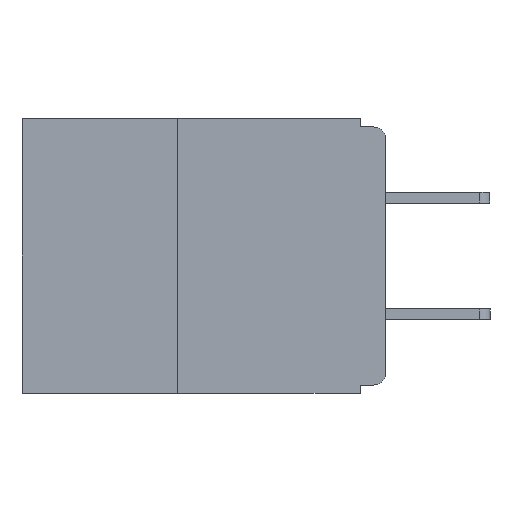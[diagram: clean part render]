
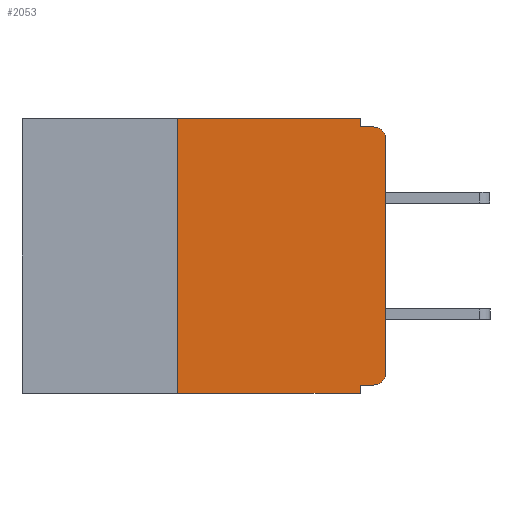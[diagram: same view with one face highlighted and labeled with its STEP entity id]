
A CAD part, left-side view. The second image highlights one B-rep face of the part: STEP entity #2053.
In plain terms, the highlighted planar face has unit normal (-1, 0, 0).
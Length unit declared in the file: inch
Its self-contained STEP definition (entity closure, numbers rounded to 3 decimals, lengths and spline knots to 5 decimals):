
#310 = DIRECTION ( 'NONE',  ( 0., 0., -1. ) ) ;
#402 = LINE ( 'NONE', #18275, #13644 ) ;
#642 = CIRCLE ( 'NONE', #13474, 0.015 ) ;
#1498 = AXIS2_PLACEMENT_3D ( 'NONE', #13234, #32510, #16109 ) ;
#2053 = ADVANCED_FACE ( 'NONE', ( #9263 ), #13210, .F. ) ;
#2341 = LINE ( 'NONE', #31891, #8912 ) ;
#2536 = ORIENTED_EDGE ( 'NONE', *, *, #6000, .F. ) ;
#2590 = ORIENTED_EDGE ( 'NONE', *, *, #15401, .F. ) ;
#2752 = CARTESIAN_POINT ( 'NONE',  ( 0., 0.25, -0.33 ) ) ;
#2807 = EDGE_CURVE ( 'NONE', #19424, #23672, #13187, .T. ) ;
#2842 = DIRECTION ( 'NONE',  ( 0., -1., 0. ) ) ;
#2897 = VERTEX_POINT ( 'NONE', #19834 ) ;
#3259 = VERTEX_POINT ( 'NONE', #11582 ) ;
#3335 = CARTESIAN_POINT ( 'NONE',  ( 0., 0., -0.305 ) ) ;
#3467 = CARTESIAN_POINT ( 'NONE',  ( 0., 0.437, -0.33 ) ) ;
#3662 = VERTEX_POINT ( 'NONE', #31116 ) ;
#3770 = LINE ( 'NONE', #13402, #25212 ) ;
#5061 = CARTESIAN_POINT ( 'NONE',  ( 0., 0.031, 0. ) ) ;
#5677 = EDGE_CURVE ( 'NONE', #13860, #12004, #34432, .T. ) ;
#6000 = EDGE_CURVE ( 'NONE', #2897, #26076, #16942, .T. ) ;
#6539 = ORIENTED_EDGE ( 'NONE', *, *, #5677, .T. ) ;
#6686 = EDGE_CURVE ( 'NONE', #26076, #3662, #2341, .T. ) ;
#7428 = LINE ( 'NONE', #5061, #35786 ) ;
#8818 = CARTESIAN_POINT ( 'NONE',  ( 0., 0.25, 0. ) ) ;
#8912 = VECTOR ( 'NONE', #31940, 39.37008 ) ;
#9180 = VERTEX_POINT ( 'NONE', #24794 ) ;
#9263 = FACE_OUTER_BOUND ( 'NONE', #31676, .T. ) ;
#9304 = ORIENTED_EDGE ( 'NONE', *, *, #29555, .F. ) ;
#9795 = EDGE_CURVE ( 'NONE', #3259, #20305, #7428, .T. ) ;
#10365 = EDGE_CURVE ( 'NONE', #19424, #3662, #18882, .T. ) ;
#11582 = CARTESIAN_POINT ( 'NONE',  ( 0., 0.031, 0. ) ) ;
#12004 = VERTEX_POINT ( 'NONE', #19621 ) ;
#12491 = EDGE_CURVE ( 'NONE', #12004, #9180, #22993, .T. ) ;
#13187 = LINE ( 'NONE', #21651, #27131 ) ;
#13210 = PLANE ( 'NONE',  #24238 ) ;
#13234 = CARTESIAN_POINT ( 'NONE',  ( 0., 0.015, -0.025 ) ) ;
#13293 = DIRECTION ( 'NONE',  ( 0., 0., -1. ) ) ;
#13402 = CARTESIAN_POINT ( 'NONE',  ( 0., 0., -0.01 ) ) ;
#13474 = AXIS2_PLACEMENT_3D ( 'NONE', #33590, #17268, #310 ) ;
#13644 = VECTOR ( 'NONE', #31937, 39.37008 ) ;
#13733 = CARTESIAN_POINT ( 'NONE',  ( 0., 0.031, -0.32 ) ) ;
#13793 = CARTESIAN_POINT ( 'NONE',  ( 0., 0.437, 0. ) ) ;
#13860 = VERTEX_POINT ( 'NONE', #3335 ) ;
#14135 = CARTESIAN_POINT ( 'NONE',  ( 0., 0., 0. ) ) ;
#14149 = DIRECTION ( 'NONE',  ( 1., 0., 0. ) ) ;
#15401 = EDGE_CURVE ( 'NONE', #20305, #9180, #3770, .T. ) ;
#16070 = ORIENTED_EDGE ( 'NONE', *, *, #9795, .F. ) ;
#16109 = DIRECTION ( 'NONE',  ( 0., 0., -1. ) ) ;
#16942 = LINE ( 'NONE', #16983, #30649 ) ;
#16983 = CARTESIAN_POINT ( 'NONE',  ( 0., 0., -0.32 ) ) ;
#17268 = DIRECTION ( 'NONE',  ( -1., 0., 0. ) ) ;
#17393 = DIRECTION ( 'NONE',  ( 0., 1., 0. ) ) ;
#17969 = VECTOR ( 'NONE', #2842, 39.37008 ) ;
#18275 = CARTESIAN_POINT ( 'NONE',  ( 0., 0.437, 0. ) ) ;
#18882 = LINE ( 'NONE', #3467, #17969 ) ;
#19424 = VERTEX_POINT ( 'NONE', #2752 ) ;
#19621 = CARTESIAN_POINT ( 'NONE',  ( 0., 0., -0.025 ) ) ;
#19834 = CARTESIAN_POINT ( 'NONE',  ( 0., 0.015, -0.32 ) ) ;
#20305 = VERTEX_POINT ( 'NONE', #20902 ) ;
#20685 = DIRECTION ( 'NONE',  ( 0., 0., 1. ) ) ;
#20902 = CARTESIAN_POINT ( 'NONE',  ( 0., 0.031, -0.01 ) ) ;
#20913 = VECTOR ( 'NONE', #20685, 39.37008 ) ;
#21651 = CARTESIAN_POINT ( 'NONE',  ( 0., 0.25, -0.33 ) ) ;
#21721 = DIRECTION ( 'NONE',  ( 0., 0., 1. ) ) ;
#21887 = DIRECTION ( 'NONE',  ( 0., 0., -1. ) ) ;
#22993 = CIRCLE ( 'NONE', #1498, 0.015 ) ;
#23672 = VERTEX_POINT ( 'NONE', #8818 ) ;
#24238 = AXIS2_PLACEMENT_3D ( 'NONE', #13793, #14149, #13293 ) ;
#24781 = ORIENTED_EDGE ( 'NONE', *, *, #6686, .F. ) ;
#24794 = CARTESIAN_POINT ( 'NONE',  ( 0., 0.015, -0.01 ) ) ;
#25212 = VECTOR ( 'NONE', #27283, 39.37008 ) ;
#26038 = ORIENTED_EDGE ( 'NONE', *, *, #10365, .T. ) ;
#26076 = VERTEX_POINT ( 'NONE', #13733 ) ;
#26886 = ORIENTED_EDGE ( 'NONE', *, *, #32274, .T. ) ;
#27131 = VECTOR ( 'NONE', #21721, 39.37008 ) ;
#27283 = DIRECTION ( 'NONE',  ( 0., -1., 0. ) ) ;
#28262 = ORIENTED_EDGE ( 'NONE', *, *, #12491, .T. ) ;
#29555 = EDGE_CURVE ( 'NONE', #23672, #3259, #402, .T. ) ;
#30166 = ORIENTED_EDGE ( 'NONE', *, *, #2807, .F. ) ;
#30649 = VECTOR ( 'NONE', #17393, 39.37008 ) ;
#31116 = CARTESIAN_POINT ( 'NONE',  ( 0., 0.031, -0.33 ) ) ;
#31676 = EDGE_LOOP ( 'NONE', ( #6539, #28262, #2590, #16070, #9304, #30166, #26038, #24781, #2536, #26886 ) ) ;
#31891 = CARTESIAN_POINT ( 'NONE',  ( 0., 0.031, -0.33 ) ) ;
#31937 = DIRECTION ( 'NONE',  ( 0., -1., 0. ) ) ;
#31940 = DIRECTION ( 'NONE',  ( 0., 0., -1. ) ) ;
#32274 = EDGE_CURVE ( 'NONE', #2897, #13860, #642, .T. ) ;
#32510 = DIRECTION ( 'NONE',  ( -1., 0., 0. ) ) ;
#33590 = CARTESIAN_POINT ( 'NONE',  ( 0., 0.015, -0.305 ) ) ;
#34432 = LINE ( 'NONE', #14135, #20913 ) ;
#35786 = VECTOR ( 'NONE', #21887, 39.37008 ) ;
